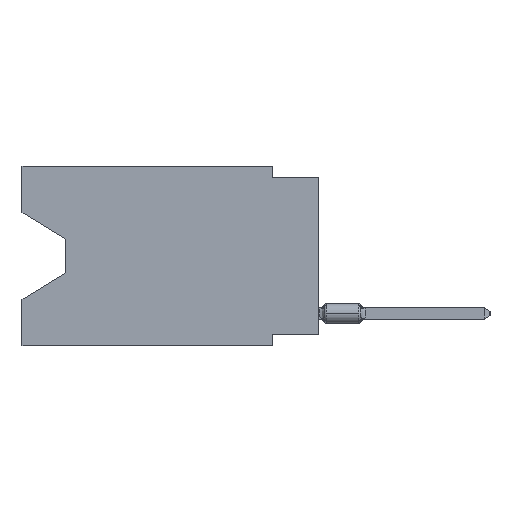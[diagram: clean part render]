
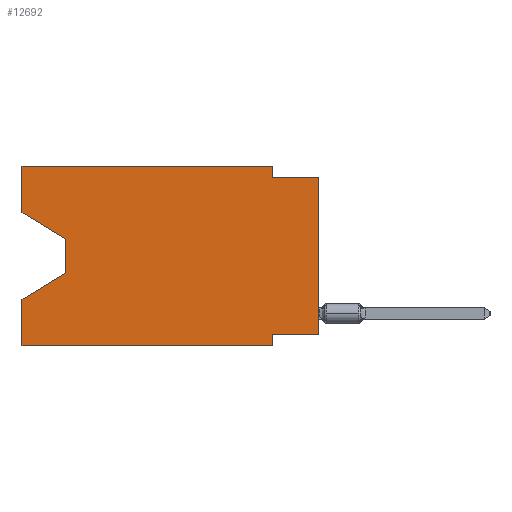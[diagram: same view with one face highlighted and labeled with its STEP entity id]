
A CAD part, left-side view. The second image highlights one B-rep face of the part: STEP entity #12692.
In plain terms, the highlighted planar face has unit normal (-1, 0, 0).
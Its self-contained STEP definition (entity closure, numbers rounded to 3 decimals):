
#92 = VERTEX_POINT ( 'NONE', #33454 ) ;
#215 = LINE ( 'NONE', #8136, #45353 ) ;
#1465 = ORIENTED_EDGE ( 'NONE', *, *, #33521, .F. ) ;
#1624 = LINE ( 'NONE', #34402, #21561 ) ;
#2411 = ORIENTED_EDGE ( 'NONE', *, *, #26981, .T. ) ;
#2957 = VERTEX_POINT ( 'NONE', #30004 ) ;
#3239 = CARTESIAN_POINT ( 'NONE',  ( 0., 16.383, -7.36 ) ) ;
#3691 = ORIENTED_EDGE ( 'NONE', *, *, #50345, .F. ) ;
#4169 = CARTESIAN_POINT ( 'NONE',  ( 0., 16.383, -2.546 ) ) ;
#4592 = CARTESIAN_POINT ( 'NONE',  ( 0., 13.97, -5.893 ) ) ;
#4654 = CARTESIAN_POINT ( 'NONE',  ( 0., 0., -0.635 ) ) ;
#6467 = CARTESIAN_POINT ( 'NONE',  ( 0., 16.383, 0. ) ) ;
#7249 = LINE ( 'NONE', #32401, #19688 ) ;
#7250 = EDGE_CURVE ( 'NONE', #30040, #31361, #18342, .T. ) ;
#8136 = CARTESIAN_POINT ( 'NONE',  ( 0., 0., -9.271 ) ) ;
#9304 = ORIENTED_EDGE ( 'NONE', *, *, #53296, .F. ) ;
#10117 = ORIENTED_EDGE ( 'NONE', *, *, #32698, .T. ) ;
#10831 = CARTESIAN_POINT ( 'NONE',  ( 0., 2.54, 0. ) ) ;
#11066 = ORIENTED_EDGE ( 'NONE', *, *, #7250, .F. ) ;
#11231 = VECTOR ( 'NONE', #25485, 1000. ) ;
#12692 = ADVANCED_FACE ( 'NONE', ( #29730 ), #13866, .F. ) ;
#13103 = CARTESIAN_POINT ( 'NONE',  ( 0., 16.383, -9.906 ) ) ;
#13216 = VECTOR ( 'NONE', #47118, 1000. ) ;
#13604 = EDGE_CURVE ( 'NONE', #23008, #25248, #14299, .T. ) ;
#13866 = PLANE ( 'NONE',  #38558 ) ;
#14299 = LINE ( 'NONE', #22243, #32835 ) ;
#16168 = VERTEX_POINT ( 'NONE', #4654 ) ;
#16648 = CARTESIAN_POINT ( 'NONE',  ( 0., 13.97, -4.013 ) ) ;
#17941 = EDGE_CURVE ( 'NONE', #33256, #19391, #1624, .T. ) ;
#17990 = DIRECTION ( 'NONE',  ( 1., 0., 0. ) ) ;
#18342 = LINE ( 'NONE', #42318, #49108 ) ;
#19391 = VERTEX_POINT ( 'NONE', #3239 ) ;
#19688 = VECTOR ( 'NONE', #23970, 1000. ) ;
#20062 = CARTESIAN_POINT ( 'NONE',  ( 0., 2.54, -9.271 ) ) ;
#21124 = LINE ( 'NONE', #37736, #11231 ) ;
#21561 = VECTOR ( 'NONE', #22968, 1000. ) ;
#21763 = EDGE_CURVE ( 'NONE', #92, #46671, #46309, .T. ) ;
#22079 = CARTESIAN_POINT ( 'NONE',  ( 0., 2.54, 0. ) ) ;
#22093 = CARTESIAN_POINT ( 'NONE',  ( 0., 16.383, 0. ) ) ;
#22243 = CARTESIAN_POINT ( 'NONE',  ( 0., 16.383, 0. ) ) ;
#22764 = CARTESIAN_POINT ( 'NONE',  ( 0., 16.383, -9.906 ) ) ;
#22968 = DIRECTION ( 'NONE',  ( 0., 0., 1. ) ) ;
#23008 = VERTEX_POINT ( 'NONE', #40245 ) ;
#23659 = CARTESIAN_POINT ( 'NONE',  ( 0., 13.97, -5.893 ) ) ;
#23917 = VECTOR ( 'NONE', #27518, 1000. ) ;
#23970 = DIRECTION ( 'NONE',  ( 0., -1., 0. ) ) ;
#24722 = LINE ( 'NONE', #22764, #37896 ) ;
#24759 = EDGE_LOOP ( 'NONE', ( #10117, #53381, #47697, #41993, #2411, #11066, #3691, #32357, #51890, #9304, #48231, #1465 ) ) ;
#25248 = VERTEX_POINT ( 'NONE', #22079 ) ;
#25485 = DIRECTION ( 'NONE',  ( 0., 0., 1. ) ) ;
#26261 = DIRECTION ( 'NONE',  ( 0., 0., -1. ) ) ;
#26981 = EDGE_CURVE ( 'NONE', #33256, #31361, #24722, .T. ) ;
#27518 = DIRECTION ( 'NONE',  ( 0., 0., -1. ) ) ;
#29291 = CARTESIAN_POINT ( 'NONE',  ( 0., 2.54, -0.635 ) ) ;
#29730 = FACE_OUTER_BOUND ( 'NONE', #24759, .T. ) ;
#29975 = DIRECTION ( 'NONE',  ( 0., 1., 0. ) ) ;
#30004 = CARTESIAN_POINT ( 'NONE',  ( 0., 16.383, -2.546 ) ) ;
#30040 = VERTEX_POINT ( 'NONE', #20062 ) ;
#31361 = VERTEX_POINT ( 'NONE', #31857 ) ;
#31857 = CARTESIAN_POINT ( 'NONE',  ( 0., 2.54, -9.906 ) ) ;
#32357 = ORIENTED_EDGE ( 'NONE', *, *, #48355, .T. ) ;
#32401 = CARTESIAN_POINT ( 'NONE',  ( 0., 0., -0.635 ) ) ;
#32698 = EDGE_CURVE ( 'NONE', #2957, #92, #45645, .T. ) ;
#32835 = VECTOR ( 'NONE', #38850, 1000. ) ;
#33256 = VERTEX_POINT ( 'NONE', #13103 ) ;
#33279 = DIRECTION ( 'NONE',  ( 0., 0., -1. ) ) ;
#33454 = CARTESIAN_POINT ( 'NONE',  ( 0., 13.97, -4.013 ) ) ;
#33521 = EDGE_CURVE ( 'NONE', #2957, #23008, #43049, .T. ) ;
#34402 = CARTESIAN_POINT ( 'NONE',  ( 0., 16.383, 0. ) ) ;
#34470 = DIRECTION ( 'NONE',  ( 0., -1., 0. ) ) ;
#37374 = LINE ( 'NONE', #4592, #51726 ) ;
#37736 = CARTESIAN_POINT ( 'NONE',  ( 0., 0., 0. ) ) ;
#37896 = VECTOR ( 'NONE', #34470, 1000. ) ;
#38558 = AXIS2_PLACEMENT_3D ( 'NONE', #22093, #17990, #50131 ) ;
#38850 = DIRECTION ( 'NONE',  ( 0., -1., 0. ) ) ;
#38934 = EDGE_CURVE ( 'NONE', #51074, #16168, #7249, .T. ) ;
#39238 = EDGE_CURVE ( 'NONE', #46671, #19391, #37374, .T. ) ;
#40245 = CARTESIAN_POINT ( 'NONE',  ( 0., 16.383, 0. ) ) ;
#41704 = DIRECTION ( 'NONE',  ( 0., 0.855, -0.519 ) ) ;
#41993 = ORIENTED_EDGE ( 'NONE', *, *, #17941, .F. ) ;
#42318 = CARTESIAN_POINT ( 'NONE',  ( 0., 2.54, -9.906 ) ) ;
#43049 = LINE ( 'NONE', #6467, #13216 ) ;
#44642 = VERTEX_POINT ( 'NONE', #51254 ) ;
#44687 = VECTOR ( 'NONE', #33279, 1000. ) ;
#45353 = VECTOR ( 'NONE', #29975, 1000. ) ;
#45645 = LINE ( 'NONE', #4169, #47935 ) ;
#46309 = LINE ( 'NONE', #16648, #44687 ) ;
#46671 = VERTEX_POINT ( 'NONE', #23659 ) ;
#47118 = DIRECTION ( 'NONE',  ( 0., 0., 1. ) ) ;
#47697 = ORIENTED_EDGE ( 'NONE', *, *, #39238, .T. ) ;
#47935 = VECTOR ( 'NONE', #53783, 1000. ) ;
#48178 = LINE ( 'NONE', #10831, #23917 ) ;
#48231 = ORIENTED_EDGE ( 'NONE', *, *, #13604, .F. ) ;
#48355 = EDGE_CURVE ( 'NONE', #44642, #16168, #21124, .T. ) ;
#49108 = VECTOR ( 'NONE', #26261, 1000. ) ;
#50131 = DIRECTION ( 'NONE',  ( 0., 0., -1. ) ) ;
#50345 = EDGE_CURVE ( 'NONE', #44642, #30040, #215, .T. ) ;
#51074 = VERTEX_POINT ( 'NONE', #29291 ) ;
#51254 = CARTESIAN_POINT ( 'NONE',  ( 0., 0., -9.271 ) ) ;
#51726 = VECTOR ( 'NONE', #41704, 1000. ) ;
#51890 = ORIENTED_EDGE ( 'NONE', *, *, #38934, .F. ) ;
#53296 = EDGE_CURVE ( 'NONE', #25248, #51074, #48178, .T. ) ;
#53381 = ORIENTED_EDGE ( 'NONE', *, *, #21763, .T. ) ;
#53783 = DIRECTION ( 'NONE',  ( 0., -0.855, -0.519 ) ) ;
